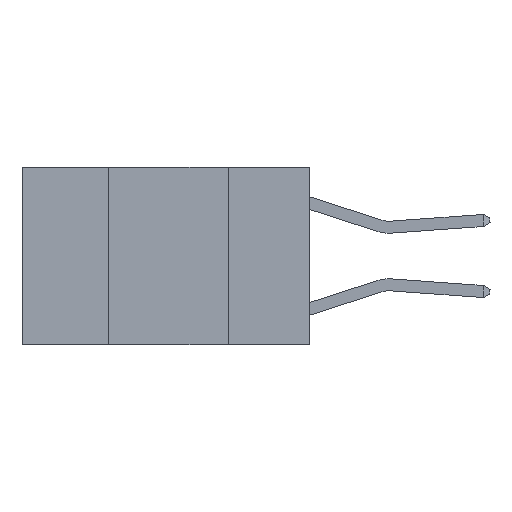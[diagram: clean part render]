
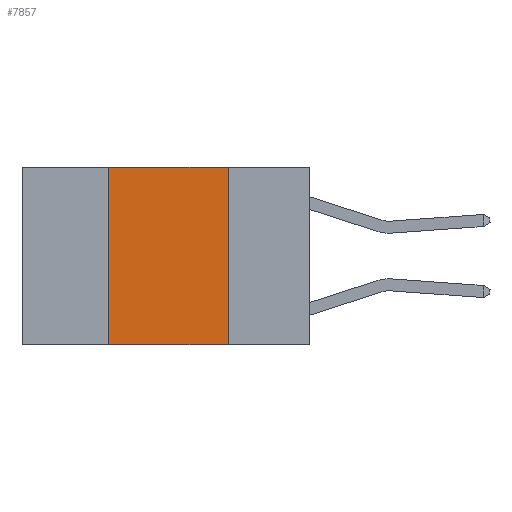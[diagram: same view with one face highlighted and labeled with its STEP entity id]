
A CAD part, left-side view. The second image highlights one B-rep face of the part: STEP entity #7857.
In plain terms, the highlighted planar face has unit normal (-1, 0, 0).
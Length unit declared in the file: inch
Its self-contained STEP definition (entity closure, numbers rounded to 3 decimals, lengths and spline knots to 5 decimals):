
#19 = EDGE_CURVE ( 'NONE', #19017, #11747, #7182, .T. ) ;
#596 = CARTESIAN_POINT ( 'NONE',  ( 0., 0.6, 0. ) ) ;
#770 = CARTESIAN_POINT ( 'NONE',  ( 0., 0.17, -0.37 ) ) ;
#1086 = ORIENTED_EDGE ( 'NONE', *, *, #19, .F. ) ;
#1339 = CARTESIAN_POINT ( 'NONE',  ( 0., 0.42, -0.37 ) ) ;
#2252 = DIRECTION ( 'NONE',  ( 1., 0., 0. ) ) ;
#3147 = CARTESIAN_POINT ( 'NONE',  ( 0., 0.6, -0.37 ) ) ;
#5283 = VERTEX_POINT ( 'NONE', #12221 ) ;
#7068 = CARTESIAN_POINT ( 'NONE',  ( 0., 0.17, 0. ) ) ;
#7165 = CARTESIAN_POINT ( 'NONE',  ( 0., 0.6, 0. ) ) ;
#7182 = LINE ( 'NONE', #7068, #19437 ) ;
#7525 = FACE_OUTER_BOUND ( 'NONE', #19492, .T. ) ;
#7857 = ADVANCED_FACE ( 'NONE', ( #7525 ), #19627, .F. ) ;
#8004 = EDGE_CURVE ( 'NONE', #11381, #11747, #11683, .T. ) ;
#8014 = CARTESIAN_POINT ( 'NONE',  ( 0., 0.42, 0. ) ) ;
#8162 = EDGE_CURVE ( 'NONE', #5283, #19017, #12353, .T. ) ;
#9600 = DIRECTION ( 'NONE',  ( 0., 0., 1. ) ) ;
#10462 = DIRECTION ( 'NONE',  ( 0., 0., -1. ) ) ;
#10608 = VECTOR ( 'NONE', #18492, 39.37008 ) ;
#11342 = VECTOR ( 'NONE', #11905, 39.37008 ) ;
#11381 = VERTEX_POINT ( 'NONE', #1339 ) ;
#11683 = LINE ( 'NONE', #3147, #10608 ) ;
#11747 = VERTEX_POINT ( 'NONE', #770 ) ;
#11905 = DIRECTION ( 'NONE',  ( 0., -1., 0. ) ) ;
#12221 = CARTESIAN_POINT ( 'NONE',  ( 0., 0.42, 0. ) ) ;
#12353 = LINE ( 'NONE', #7165, #11342 ) ;
#12710 = DIRECTION ( 'NONE',  ( 0., 0., -1. ) ) ;
#15299 = VECTOR ( 'NONE', #9600, 39.37008 ) ;
#16773 = LINE ( 'NONE', #8014, #15299 ) ;
#17007 = AXIS2_PLACEMENT_3D ( 'NONE', #596, #2252, #12710 ) ;
#17966 = ORIENTED_EDGE ( 'NONE', *, *, #18238, .F. ) ;
#18238 = EDGE_CURVE ( 'NONE', #11381, #5283, #16773, .T. ) ;
#18312 = ORIENTED_EDGE ( 'NONE', *, *, #8162, .F. ) ;
#18492 = DIRECTION ( 'NONE',  ( 0., -1., 0. ) ) ;
#18676 = CARTESIAN_POINT ( 'NONE',  ( 0., 0.17, 0. ) ) ;
#19017 = VERTEX_POINT ( 'NONE', #18676 ) ;
#19437 = VECTOR ( 'NONE', #10462, 39.37008 ) ;
#19492 = EDGE_LOOP ( 'NONE', ( #1086, #18312, #17966, #21643 ) ) ;
#19627 = PLANE ( 'NONE',  #17007 ) ;
#21643 = ORIENTED_EDGE ( 'NONE', *, *, #8004, .T. ) ;
